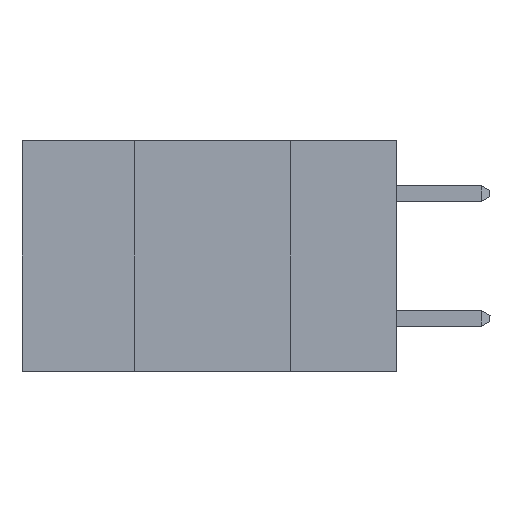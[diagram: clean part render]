
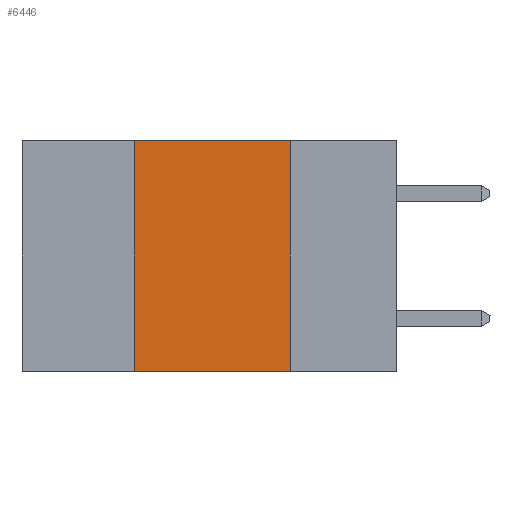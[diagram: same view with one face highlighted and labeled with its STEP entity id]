
A CAD part, left-side view. The second image highlights one B-rep face of the part: STEP entity #6446.
In plain terms, the highlighted planar face has unit normal (-1, 0, 0).
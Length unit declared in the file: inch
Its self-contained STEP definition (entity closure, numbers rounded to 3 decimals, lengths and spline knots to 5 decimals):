
#296 = CARTESIAN_POINT ( 'NONE',  ( 0., 0.6, 0. ) ) ;
#951 = CARTESIAN_POINT ( 'NONE',  ( 0., 0.42, -0.37 ) ) ;
#1171 = AXIS2_PLACEMENT_3D ( 'NONE', #296, #11823, #17578 ) ;
#1944 = DIRECTION ( 'NONE',  ( 0., -1., 0. ) ) ;
#1998 = CARTESIAN_POINT ( 'NONE',  ( 0., 0.17, -0.37 ) ) ;
#2693 = VERTEX_POINT ( 'NONE', #951 ) ;
#3109 = EDGE_CURVE ( 'NONE', #2693, #10031, #21090, .T. ) ;
#4327 = VECTOR ( 'NONE', #15687, 39.37008 ) ;
#5593 = EDGE_CURVE ( 'NONE', #11469, #10031, #8718, .T. ) ;
#6446 = ADVANCED_FACE ( 'NONE', ( #13775 ), #14091, .F. ) ;
#6491 = EDGE_CURVE ( 'NONE', #2693, #17385, #16702, .T. ) ;
#7709 = ORIENTED_EDGE ( 'NONE', *, *, #6491, .F. ) ;
#8718 = LINE ( 'NONE', #13239, #16743 ) ;
#8782 = CARTESIAN_POINT ( 'NONE',  ( 0., 0.6, -0.37 ) ) ;
#9457 = VECTOR ( 'NONE', #1944, 39.37008 ) ;
#9667 = ORIENTED_EDGE ( 'NONE', *, *, #3109, .T. ) ;
#9778 = DIRECTION ( 'NONE',  ( 0., 0., -1. ) ) ;
#10031 = VERTEX_POINT ( 'NONE', #1998 ) ;
#10711 = EDGE_CURVE ( 'NONE', #17385, #11469, #11605, .T. ) ;
#11455 = ORIENTED_EDGE ( 'NONE', *, *, #10711, .F. ) ;
#11469 = VERTEX_POINT ( 'NONE', #13575 ) ;
#11605 = LINE ( 'NONE', #17429, #9457 ) ;
#11823 = DIRECTION ( 'NONE',  ( 1., 0., 0. ) ) ;
#12779 = CARTESIAN_POINT ( 'NONE',  ( 0., 0.42, 0. ) ) ;
#13229 = EDGE_LOOP ( 'NONE', ( #18445, #11455, #7709, #9667 ) ) ;
#13239 = CARTESIAN_POINT ( 'NONE',  ( 0., 0.17, 0. ) ) ;
#13575 = CARTESIAN_POINT ( 'NONE',  ( 0., 0.17, 0. ) ) ;
#13775 = FACE_OUTER_BOUND ( 'NONE', #13229, .T. ) ;
#14091 = PLANE ( 'NONE',  #1171 ) ;
#15687 = DIRECTION ( 'NONE',  ( 0., -1., 0. ) ) ;
#16702 = LINE ( 'NONE', #19242, #20783 ) ;
#16743 = VECTOR ( 'NONE', #9778, 39.37008 ) ;
#17385 = VERTEX_POINT ( 'NONE', #12779 ) ;
#17429 = CARTESIAN_POINT ( 'NONE',  ( 0., 0.6, 0. ) ) ;
#17578 = DIRECTION ( 'NONE',  ( 0., 0., -1. ) ) ;
#18445 = ORIENTED_EDGE ( 'NONE', *, *, #5593, .F. ) ;
#19242 = CARTESIAN_POINT ( 'NONE',  ( 0., 0.42, 0. ) ) ;
#19456 = DIRECTION ( 'NONE',  ( 0., 0., 1. ) ) ;
#20783 = VECTOR ( 'NONE', #19456, 39.37008 ) ;
#21090 = LINE ( 'NONE', #8782, #4327 ) ;
